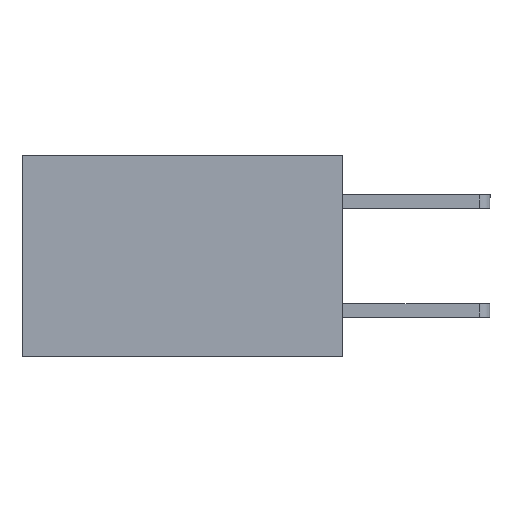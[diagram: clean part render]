
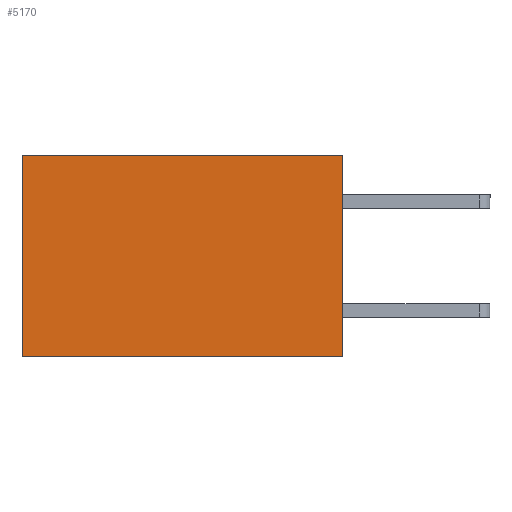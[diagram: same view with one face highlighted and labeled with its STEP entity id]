
A CAD part, left-side view. The second image highlights one B-rep face of the part: STEP entity #5170.
In plain terms, the highlighted planar face has unit normal (-1, 0, 0).
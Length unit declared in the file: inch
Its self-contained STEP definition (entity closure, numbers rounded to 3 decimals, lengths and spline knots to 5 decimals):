
#106 = ORIENTED_EDGE ( 'NONE', *, *, #5856, .F. ) ;
#285 = EDGE_LOOP ( 'NONE', ( #2769, #1389, #106, #913 ) ) ;
#381 = VERTEX_POINT ( 'NONE', #6947 ) ;
#829 = CARTESIAN_POINT ( 'NONE',  ( 0.277, 0., -0.37 ) ) ;
#850 = LINE ( 'NONE', #7219, #7296 ) ;
#913 = ORIENTED_EDGE ( 'NONE', *, *, #1920, .T. ) ;
#1389 = ORIENTED_EDGE ( 'NONE', *, *, #2958, .F. ) ;
#1550 = VECTOR ( 'NONE', #7270, 39.37008 ) ;
#1920 = EDGE_CURVE ( 'NONE', #2285, #3006, #850, .T. ) ;
#2285 = VERTEX_POINT ( 'NONE', #6840 ) ;
#2739 = CARTESIAN_POINT ( 'NONE',  ( 0.277, 0.59, -0.37 ) ) ;
#2766 = DIRECTION ( 'NONE',  ( 0., 0., -1. ) ) ;
#2769 = ORIENTED_EDGE ( 'NONE', *, *, #7930, .T. ) ;
#2958 = EDGE_CURVE ( 'NONE', #7789, #381, #6339, .T. ) ;
#3006 = VERTEX_POINT ( 'NONE', #3776 ) ;
#3305 = CARTESIAN_POINT ( 'NONE',  ( 0.277, 0., -0.37 ) ) ;
#3679 = AXIS2_PLACEMENT_3D ( 'NONE', #4631, #4601, #4610 ) ;
#3776 = CARTESIAN_POINT ( 'NONE',  ( 0.277, 0.59, 0. ) ) ;
#4343 = LINE ( 'NONE', #2739, #5785 ) ;
#4559 = DIRECTION ( 'NONE',  ( 0., 1., 0. ) ) ;
#4601 = DIRECTION ( 'NONE',  ( 1., 0., 0. ) ) ;
#4610 = DIRECTION ( 'NONE',  ( 0., 0., -1. ) ) ;
#4631 = CARTESIAN_POINT ( 'NONE',  ( 0.277, 0., -0.37 ) ) ;
#5170 = ADVANCED_FACE ( 'NONE', ( #6590 ), #6183, .F. ) ;
#5408 = DIRECTION ( 'NONE',  ( 0., 0., -1. ) ) ;
#5415 = CARTESIAN_POINT ( 'NONE',  ( 0.277, 0., -0.37 ) ) ;
#5724 = VECTOR ( 'NONE', #5408, 39.37008 ) ;
#5785 = VECTOR ( 'NONE', #2766, 39.37008 ) ;
#5856 = EDGE_CURVE ( 'NONE', #2285, #7789, #7120, .T. ) ;
#6183 = PLANE ( 'NONE',  #3679 ) ;
#6339 = LINE ( 'NONE', #829, #1550 ) ;
#6590 = FACE_OUTER_BOUND ( 'NONE', #285, .T. ) ;
#6840 = CARTESIAN_POINT ( 'NONE',  ( 0.277, 0., 0. ) ) ;
#6947 = CARTESIAN_POINT ( 'NONE',  ( 0.277, 0.59, -0.37 ) ) ;
#7120 = LINE ( 'NONE', #5415, #5724 ) ;
#7219 = CARTESIAN_POINT ( 'NONE',  ( 0.277, 0., 0. ) ) ;
#7270 = DIRECTION ( 'NONE',  ( 0., 1., 0. ) ) ;
#7296 = VECTOR ( 'NONE', #4559, 39.37008 ) ;
#7789 = VERTEX_POINT ( 'NONE', #3305 ) ;
#7930 = EDGE_CURVE ( 'NONE', #3006, #381, #4343, .T. ) ;
